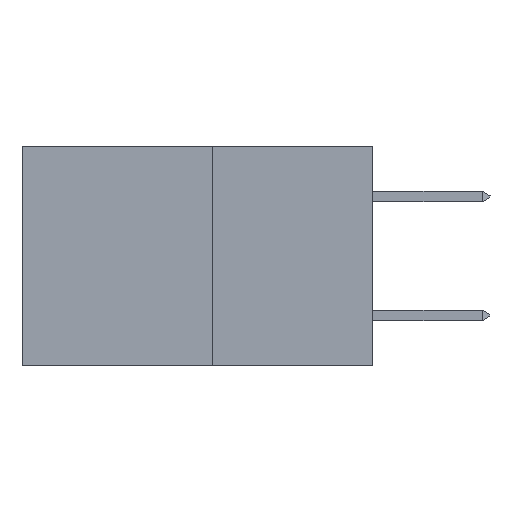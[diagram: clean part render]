
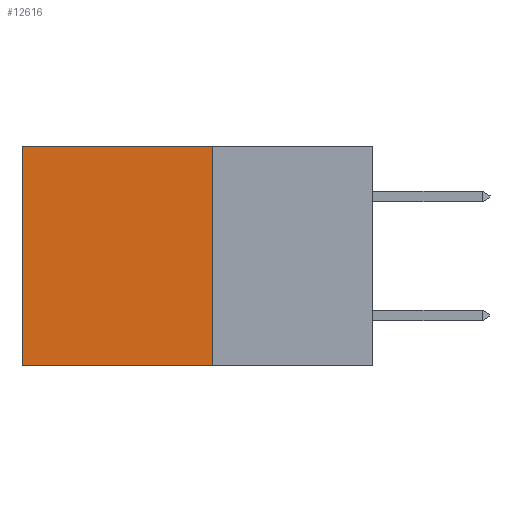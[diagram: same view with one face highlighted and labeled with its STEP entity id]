
A CAD part, left-side view. The second image highlights one B-rep face of the part: STEP entity #12616.
In plain terms, the highlighted planar face has unit normal (-1, 0, 0).
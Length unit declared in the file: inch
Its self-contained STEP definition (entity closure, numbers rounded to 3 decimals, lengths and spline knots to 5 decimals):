
#144 = PLANE ( 'NONE',  #3313 ) ;
#1229 = VERTEX_POINT ( 'NONE', #14629 ) ;
#1576 = EDGE_CURVE ( 'NONE', #25824, #19722, #20847, .T. ) ;
#2456 = CARTESIAN_POINT ( 'NONE',  ( 0.277, 0.27, -0.37 ) ) ;
#2566 = CARTESIAN_POINT ( 'NONE',  ( 0.277, 0.27, 0. ) ) ;
#3313 = AXIS2_PLACEMENT_3D ( 'NONE', #2456, #4767, #20445 ) ;
#4228 = VECTOR ( 'NONE', #8571, 39.37008 ) ;
#4480 = FACE_OUTER_BOUND ( 'NONE', #19194, .T. ) ;
#4767 = DIRECTION ( 'NONE',  ( 1., 0., 0. ) ) ;
#4877 = DIRECTION ( 'NONE',  ( 0., 1., 0. ) ) ;
#8278 = ORIENTED_EDGE ( 'NONE', *, *, #1576, .F. ) ;
#8571 = DIRECTION ( 'NONE',  ( 0., 0., -1. ) ) ;
#8758 = LINE ( 'NONE', #20117, #25953 ) ;
#9163 = LINE ( 'NONE', #2566, #25638 ) ;
#11055 = EDGE_CURVE ( 'NONE', #1229, #19722, #8758, .T. ) ;
#12616 = ADVANCED_FACE ( 'NONE', ( #4480 ), #144, .F. ) ;
#14311 = ORIENTED_EDGE ( 'NONE', *, *, #18745, .T. ) ;
#14629 = CARTESIAN_POINT ( 'NONE',  ( 0.277, 0.59, 0. ) ) ;
#16638 = ORIENTED_EDGE ( 'NONE', *, *, #11055, .T. ) ;
#18745 = EDGE_CURVE ( 'NONE', #19010, #1229, #9163, .T. ) ;
#19010 = VERTEX_POINT ( 'NONE', #21342 ) ;
#19194 = EDGE_LOOP ( 'NONE', ( #16638, #8278, #19306, #14311 ) ) ;
#19306 = ORIENTED_EDGE ( 'NONE', *, *, #22554, .F. ) ;
#19722 = VERTEX_POINT ( 'NONE', #28134 ) ;
#20107 = VECTOR ( 'NONE', #27175, 39.37008 ) ;
#20117 = CARTESIAN_POINT ( 'NONE',  ( 0.277, 0.59, -0.37 ) ) ;
#20445 = DIRECTION ( 'NONE',  ( 0., 0., -1. ) ) ;
#20847 = LINE ( 'NONE', #26017, #20107 ) ;
#21342 = CARTESIAN_POINT ( 'NONE',  ( 0.277, 0.27, 0. ) ) ;
#22405 = DIRECTION ( 'NONE',  ( 0., 0., -1. ) ) ;
#22554 = EDGE_CURVE ( 'NONE', #19010, #25824, #27401, .T. ) ;
#23344 = CARTESIAN_POINT ( 'NONE',  ( 0.277, 0.27, -0.37 ) ) ;
#25638 = VECTOR ( 'NONE', #4877, 39.37008 ) ;
#25824 = VERTEX_POINT ( 'NONE', #23344 ) ;
#25953 = VECTOR ( 'NONE', #22405, 39.37008 ) ;
#26017 = CARTESIAN_POINT ( 'NONE',  ( 0.277, 0.27, -0.37 ) ) ;
#27175 = DIRECTION ( 'NONE',  ( 0., 1., 0. ) ) ;
#27401 = LINE ( 'NONE', #28737, #4228 ) ;
#28134 = CARTESIAN_POINT ( 'NONE',  ( 0.277, 0.59, -0.37 ) ) ;
#28737 = CARTESIAN_POINT ( 'NONE',  ( 0.277, 0.27, -0.37 ) ) ;
